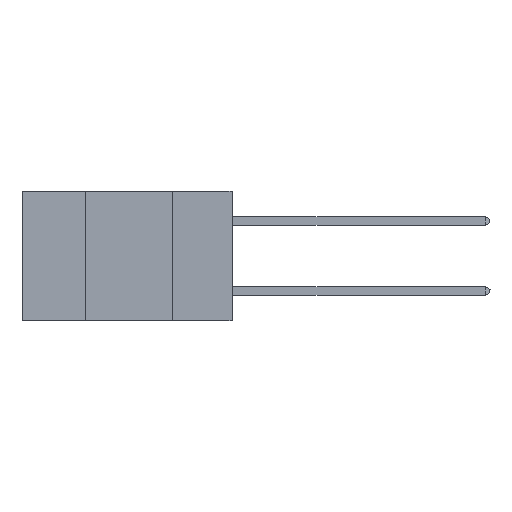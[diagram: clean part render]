
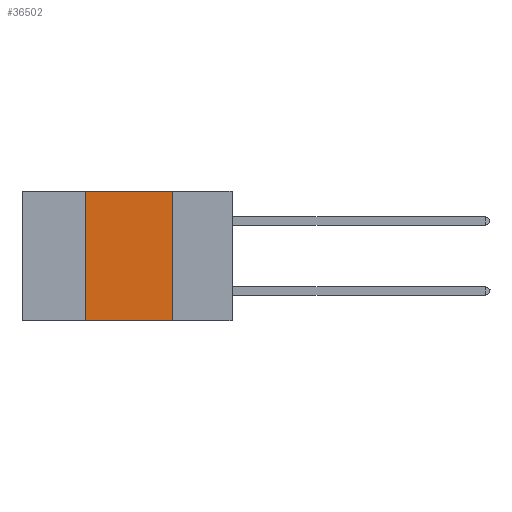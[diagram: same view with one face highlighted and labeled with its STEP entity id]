
A CAD part, left-side view. The second image highlights one B-rep face of the part: STEP entity #36502.
In plain terms, the highlighted planar face has unit normal (-1, 0, 0).
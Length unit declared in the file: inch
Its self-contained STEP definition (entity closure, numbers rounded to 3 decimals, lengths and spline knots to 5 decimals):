
#833 = CARTESIAN_POINT ( 'NONE',  ( 0., 0.17, 0. ) ) ;
#1304 = DIRECTION ( 'NONE',  ( 1., 0., 0. ) ) ;
#1347 = VECTOR ( 'NONE', #8545, 39.37008 ) ;
#1880 = EDGE_LOOP ( 'NONE', ( #31732, #26890, #3436, #15831 ) ) ;
#3436 = ORIENTED_EDGE ( 'NONE', *, *, #22703, .F. ) ;
#4008 = CARTESIAN_POINT ( 'NONE',  ( 0., 0.6, -0.37 ) ) ;
#4142 = DIRECTION ( 'NONE',  ( 0., -1., 0. ) ) ;
#4539 = CARTESIAN_POINT ( 'NONE',  ( 0., 0.42, 0. ) ) ;
#4760 = LINE ( 'NONE', #4008, #36463 ) ;
#6885 = CARTESIAN_POINT ( 'NONE',  ( 0., 0.17, 0. ) ) ;
#7526 = PLANE ( 'NONE',  #31673 ) ;
#8149 = VERTEX_POINT ( 'NONE', #4539 ) ;
#8545 = DIRECTION ( 'NONE',  ( 0., 0., 1. ) ) ;
#8962 = VERTEX_POINT ( 'NONE', #27451 ) ;
#10642 = DIRECTION ( 'NONE',  ( 0., 0., -1. ) ) ;
#11212 = LINE ( 'NONE', #833, #35477 ) ;
#11458 = CARTESIAN_POINT ( 'NONE',  ( 0., 0.42, 0. ) ) ;
#13912 = CARTESIAN_POINT ( 'NONE',  ( 0., 0.6, 0. ) ) ;
#15831 = ORIENTED_EDGE ( 'NONE', *, *, #35134, .T. ) ;
#16402 = EDGE_CURVE ( 'NONE', #39687, #20923, #11212, .T. ) ;
#20172 = LINE ( 'NONE', #11458, #1347 ) ;
#20923 = VERTEX_POINT ( 'NONE', #36870 ) ;
#21421 = FACE_OUTER_BOUND ( 'NONE', #1880, .T. ) ;
#22703 = EDGE_CURVE ( 'NONE', #8962, #8149, #20172, .T. ) ;
#25973 = VECTOR ( 'NONE', #35921, 39.37008 ) ;
#26890 = ORIENTED_EDGE ( 'NONE', *, *, #35861, .F. ) ;
#27451 = CARTESIAN_POINT ( 'NONE',  ( 0., 0.42, -0.37 ) ) ;
#31673 = AXIS2_PLACEMENT_3D ( 'NONE', #32831, #1304, #39608 ) ;
#31732 = ORIENTED_EDGE ( 'NONE', *, *, #16402, .F. ) ;
#32831 = CARTESIAN_POINT ( 'NONE',  ( 0., 0.6, 0. ) ) ;
#35134 = EDGE_CURVE ( 'NONE', #8962, #20923, #4760, .T. ) ;
#35477 = VECTOR ( 'NONE', #10642, 39.37008 ) ;
#35861 = EDGE_CURVE ( 'NONE', #8149, #39687, #39820, .T. ) ;
#35921 = DIRECTION ( 'NONE',  ( 0., -1., 0. ) ) ;
#36463 = VECTOR ( 'NONE', #4142, 39.37008 ) ;
#36502 = ADVANCED_FACE ( 'NONE', ( #21421 ), #7526, .F. ) ;
#36870 = CARTESIAN_POINT ( 'NONE',  ( 0., 0.17, -0.37 ) ) ;
#39608 = DIRECTION ( 'NONE',  ( 0., 0., -1. ) ) ;
#39687 = VERTEX_POINT ( 'NONE', #6885 ) ;
#39820 = LINE ( 'NONE', #13912, #25973 ) ;
